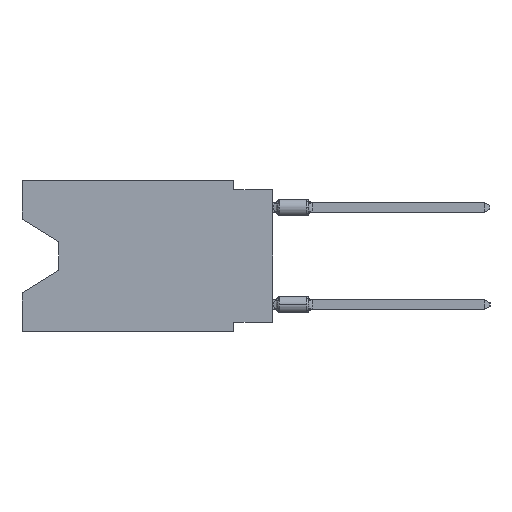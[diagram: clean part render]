
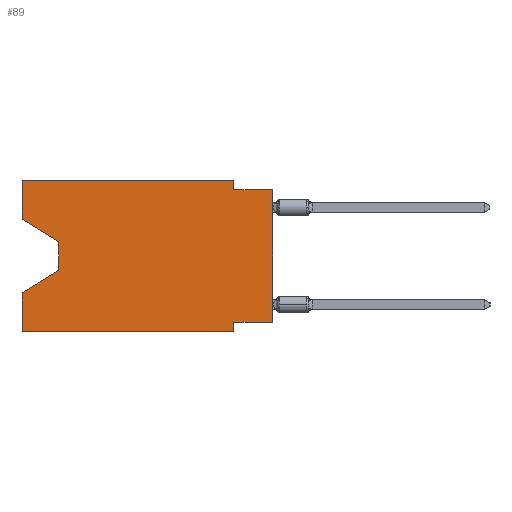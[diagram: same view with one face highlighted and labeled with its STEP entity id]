
A CAD part, left-side view. The second image highlights one B-rep face of the part: STEP entity #89.
In plain terms, the highlighted planar face has unit normal (-1, 0, 0).
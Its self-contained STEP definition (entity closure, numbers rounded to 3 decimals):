
#89 = ADVANCED_FACE ( 'NONE', ( #43964 ), #12357, .F. ) ;
#107 = DIRECTION ( 'NONE',  ( 0., 0., 1. ) ) ;
#672 = CARTESIAN_POINT ( 'NONE',  ( 0., 2.54, 0. ) ) ;
#793 = LINE ( 'NONE', #11415, #43828 ) ;
#1602 = EDGE_CURVE ( 'NONE', #33135, #29514, #46305, .T. ) ;
#2227 = CARTESIAN_POINT ( 'NONE',  ( 0., 13.97, -4.013 ) ) ;
#2512 = VERTEX_POINT ( 'NONE', #23892 ) ;
#2647 = VERTEX_POINT ( 'NONE', #35406 ) ;
#2715 = DIRECTION ( 'NONE',  ( 0., 0., -1. ) ) ;
#2821 = CARTESIAN_POINT ( 'NONE',  ( 0., 13.97, -5.893 ) ) ;
#3477 = DIRECTION ( 'NONE',  ( 0., 0., -1. ) ) ;
#3572 = LINE ( 'NONE', #46498, #9052 ) ;
#4460 = VERTEX_POINT ( 'NONE', #27060 ) ;
#4916 = AXIS2_PLACEMENT_3D ( 'NONE', #12592, #15674, #12115 ) ;
#5159 = ORIENTED_EDGE ( 'NONE', *, *, #23136, .T. ) ;
#5606 = DIRECTION ( 'NONE',  ( 0., -1., 0. ) ) ;
#6455 = EDGE_CURVE ( 'NONE', #32076, #29460, #28678, .T. ) ;
#6881 = CARTESIAN_POINT ( 'NONE',  ( 0., 2.54, -9.906 ) ) ;
#7514 = VECTOR ( 'NONE', #43523, 1000. ) ;
#8061 = EDGE_LOOP ( 'NONE', ( #15062, #29564, #5159, #32791, #24159, #22619, #34604, #30935, #44387, #38140, #40700, #28435 ) ) ;
#9052 = VECTOR ( 'NONE', #17247, 1000. ) ;
#9122 = LINE ( 'NONE', #15550, #14471 ) ;
#9959 = VECTOR ( 'NONE', #41202, 1000. ) ;
#10734 = CARTESIAN_POINT ( 'NONE',  ( 0., 16.383, 0. ) ) ;
#11415 = CARTESIAN_POINT ( 'NONE',  ( 0., 16.383, 0. ) ) ;
#12100 = DIRECTION ( 'NONE',  ( 0., -1., 0. ) ) ;
#12115 = DIRECTION ( 'NONE',  ( 0., 0., -1. ) ) ;
#12357 = PLANE ( 'NONE',  #4916 ) ;
#12480 = VERTEX_POINT ( 'NONE', #20369 ) ;
#12592 = CARTESIAN_POINT ( 'NONE',  ( 0., 16.383, 0. ) ) ;
#13666 = DIRECTION ( 'NONE',  ( 0., 0.855, -0.519 ) ) ;
#13894 = EDGE_CURVE ( 'NONE', #29460, #37954, #18948, .T. ) ;
#14471 = VECTOR ( 'NONE', #5606, 1000. ) ;
#15010 = EDGE_CURVE ( 'NONE', #33151, #37954, #46582, .T. ) ;
#15062 = ORIENTED_EDGE ( 'NONE', *, *, #45493, .T. ) ;
#15550 = CARTESIAN_POINT ( 'NONE',  ( 0., 16.383, -9.906 ) ) ;
#15674 = DIRECTION ( 'NONE',  ( 1., 0., 0. ) ) ;
#16527 = VERTEX_POINT ( 'NONE', #39906 ) ;
#16577 = CARTESIAN_POINT ( 'NONE',  ( 0., 2.54, -9.271 ) ) ;
#17247 = DIRECTION ( 'NONE',  ( 0., -1., 0. ) ) ;
#17336 = LINE ( 'NONE', #10734, #38442 ) ;
#17786 = DIRECTION ( 'NONE',  ( 0., 0., -1. ) ) ;
#18948 = LINE ( 'NONE', #33320, #24345 ) ;
#19744 = CARTESIAN_POINT ( 'NONE',  ( 0., 0., -9.271 ) ) ;
#20369 = CARTESIAN_POINT ( 'NONE',  ( 0., 16.383, 0. ) ) ;
#20729 = VECTOR ( 'NONE', #13666, 1000. ) ;
#22319 = LINE ( 'NONE', #29587, #7514 ) ;
#22619 = ORIENTED_EDGE ( 'NONE', *, *, #1602, .F. ) ;
#23136 = EDGE_CURVE ( 'NONE', #2647, #2512, #36062, .T. ) ;
#23892 = CARTESIAN_POINT ( 'NONE',  ( 0., 16.383, -7.36 ) ) ;
#24159 = ORIENTED_EDGE ( 'NONE', *, *, #26131, .T. ) ;
#24345 = VECTOR ( 'NONE', #12100, 1000. ) ;
#25175 = EDGE_CURVE ( 'NONE', #16527, #2512, #17336, .T. ) ;
#25803 = DIRECTION ( 'NONE',  ( 0., 0., 1. ) ) ;
#26131 = EDGE_CURVE ( 'NONE', #16527, #29514, #9122, .T. ) ;
#26809 = EDGE_CURVE ( 'NONE', #35668, #12480, #793, .T. ) ;
#27060 = CARTESIAN_POINT ( 'NONE',  ( 0., 13.97, -4.013 ) ) ;
#28180 = DIRECTION ( 'NONE',  ( 0., 0., 1. ) ) ;
#28435 = ORIENTED_EDGE ( 'NONE', *, *, #26809, .F. ) ;
#28678 = LINE ( 'NONE', #35793, #39184 ) ;
#29460 = VERTEX_POINT ( 'NONE', #38647 ) ;
#29514 = VERTEX_POINT ( 'NONE', #39100 ) ;
#29564 = ORIENTED_EDGE ( 'NONE', *, *, #43104, .T. ) ;
#29587 = CARTESIAN_POINT ( 'NONE',  ( 0., 16.383, -2.546 ) ) ;
#29841 = EDGE_CURVE ( 'NONE', #33151, #33135, #44737, .T. ) ;
#30297 = VECTOR ( 'NONE', #2715, 1000. ) ;
#30935 = ORIENTED_EDGE ( 'NONE', *, *, #15010, .T. ) ;
#31420 = CARTESIAN_POINT ( 'NONE',  ( 0., 0., -9.271 ) ) ;
#32076 = VERTEX_POINT ( 'NONE', #672 ) ;
#32791 = ORIENTED_EDGE ( 'NONE', *, *, #25175, .F. ) ;
#33135 = VERTEX_POINT ( 'NONE', #16577 ) ;
#33151 = VERTEX_POINT ( 'NONE', #31420 ) ;
#33320 = CARTESIAN_POINT ( 'NONE',  ( 0., 0., -0.635 ) ) ;
#33464 = VECTOR ( 'NONE', #107, 1000. ) ;
#34534 = LINE ( 'NONE', #2227, #30297 ) ;
#34604 = ORIENTED_EDGE ( 'NONE', *, *, #29841, .F. ) ;
#35054 = VECTOR ( 'NONE', #17786, 1000. ) ;
#35406 = CARTESIAN_POINT ( 'NONE',  ( 0., 13.97, -5.893 ) ) ;
#35668 = VERTEX_POINT ( 'NONE', #36161 ) ;
#35793 = CARTESIAN_POINT ( 'NONE',  ( 0., 2.54, 0. ) ) ;
#36062 = LINE ( 'NONE', #2821, #20729 ) ;
#36161 = CARTESIAN_POINT ( 'NONE',  ( 0., 16.383, -2.546 ) ) ;
#37954 = VERTEX_POINT ( 'NONE', #39857 ) ;
#38140 = ORIENTED_EDGE ( 'NONE', *, *, #6455, .F. ) ;
#38442 = VECTOR ( 'NONE', #28180, 1000. ) ;
#38647 = CARTESIAN_POINT ( 'NONE',  ( 0., 2.54, -0.635 ) ) ;
#39100 = CARTESIAN_POINT ( 'NONE',  ( 0., 2.54, -9.906 ) ) ;
#39184 = VECTOR ( 'NONE', #3477, 1000. ) ;
#39857 = CARTESIAN_POINT ( 'NONE',  ( 0., 0., -0.635 ) ) ;
#39906 = CARTESIAN_POINT ( 'NONE',  ( 0., 16.383, -9.906 ) ) ;
#40700 = ORIENTED_EDGE ( 'NONE', *, *, #46185, .F. ) ;
#41202 = DIRECTION ( 'NONE',  ( 0., 1., 0. ) ) ;
#43104 = EDGE_CURVE ( 'NONE', #4460, #2647, #34534, .T. ) ;
#43497 = CARTESIAN_POINT ( 'NONE',  ( 0., 0., 0. ) ) ;
#43523 = DIRECTION ( 'NONE',  ( 0., -0.855, -0.519 ) ) ;
#43828 = VECTOR ( 'NONE', #25803, 1000. ) ;
#43964 = FACE_OUTER_BOUND ( 'NONE', #8061, .T. ) ;
#44387 = ORIENTED_EDGE ( 'NONE', *, *, #13894, .F. ) ;
#44737 = LINE ( 'NONE', #19744, #9959 ) ;
#45493 = EDGE_CURVE ( 'NONE', #35668, #4460, #22319, .T. ) ;
#46185 = EDGE_CURVE ( 'NONE', #12480, #32076, #3572, .T. ) ;
#46305 = LINE ( 'NONE', #6881, #35054 ) ;
#46498 = CARTESIAN_POINT ( 'NONE',  ( 0., 16.383, 0. ) ) ;
#46582 = LINE ( 'NONE', #43497, #33464 ) ;
